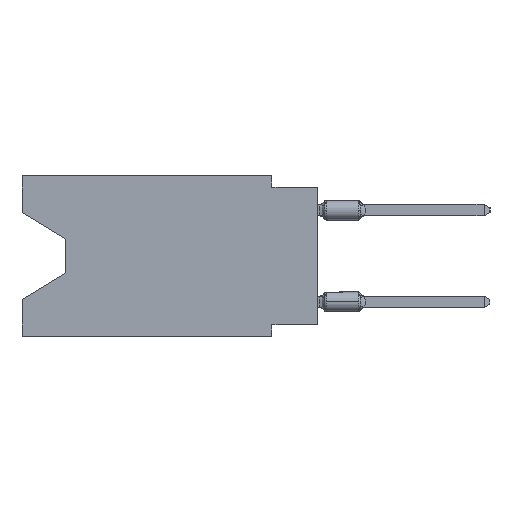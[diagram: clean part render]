
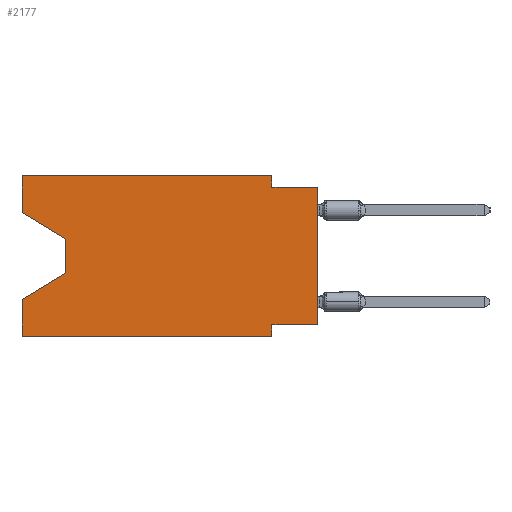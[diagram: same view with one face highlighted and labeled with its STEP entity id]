
A CAD part, left-side view. The second image highlights one B-rep face of the part: STEP entity #2177.
In plain terms, the highlighted planar face has unit normal (-1, 0, 0).
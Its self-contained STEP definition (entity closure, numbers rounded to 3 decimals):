
#264 = LINE ( 'NONE', #4096, #41204 ) ;
#921 = EDGE_CURVE ( 'NONE', #3850, #40693, #20967, .T. ) ;
#2175 = ORIENTED_EDGE ( 'NONE', *, *, #921, .F. ) ;
#2177 = ADVANCED_FACE ( 'NONE', ( #38050 ), #8898, .F. ) ;
#2750 = VERTEX_POINT ( 'NONE', #29670 ) ;
#3200 = CARTESIAN_POINT ( 'NONE',  ( 0., 16.383, 0. ) ) ;
#3461 = DIRECTION ( 'NONE',  ( 0., 0.855, -0.519 ) ) ;
#3782 = CARTESIAN_POINT ( 'NONE',  ( 0., 0., -8.255 ) ) ;
#3817 = LINE ( 'NONE', #3200, #16447 ) ;
#3850 = VERTEX_POINT ( 'NONE', #8228 ) ;
#4074 = ORIENTED_EDGE ( 'NONE', *, *, #18915, .T. ) ;
#4096 = CARTESIAN_POINT ( 'NONE',  ( 0., 0., -0.635 ) ) ;
#4331 = CARTESIAN_POINT ( 'NONE',  ( 0., 2.54, -8.89 ) ) ;
#5029 = VERTEX_POINT ( 'NONE', #3782 ) ;
#5121 = VECTOR ( 'NONE', #6302, 1000. ) ;
#5328 = EDGE_CURVE ( 'NONE', #8839, #17638, #25675, .T. ) ;
#5792 = CARTESIAN_POINT ( 'NONE',  ( 0., 16.383, 0. ) ) ;
#5820 = EDGE_LOOP ( 'NONE', ( #4074, #32551, #6760, #31467, #9528, #18816, #40151, #29738, #10410, #2175, #34779, #16425 ) ) ;
#6302 = DIRECTION ( 'NONE',  ( 0., 0., -1. ) ) ;
#6650 = CARTESIAN_POINT ( 'NONE',  ( 0., 13.97, -5.385 ) ) ;
#6760 = ORIENTED_EDGE ( 'NONE', *, *, #22581, .T. ) ;
#8009 = VECTOR ( 'NONE', #10311, 1000. ) ;
#8228 = CARTESIAN_POINT ( 'NONE',  ( 0., 2.54, 0. ) ) ;
#8285 = EDGE_CURVE ( 'NONE', #5029, #39545, #39004, .T. ) ;
#8588 = LINE ( 'NONE', #41334, #36419 ) ;
#8731 = EDGE_CURVE ( 'NONE', #36822, #3850, #16636, .T. ) ;
#8839 = VERTEX_POINT ( 'NONE', #11073 ) ;
#8898 = PLANE ( 'NONE',  #18575 ) ;
#9528 = ORIENTED_EDGE ( 'NONE', *, *, #11118, .T. ) ;
#9537 = EDGE_CURVE ( 'NONE', #40693, #39545, #264, .T. ) ;
#10311 = DIRECTION ( 'NONE',  ( 0., -1., 0. ) ) ;
#10410 = ORIENTED_EDGE ( 'NONE', *, *, #9537, .F. ) ;
#10954 = CARTESIAN_POINT ( 'NONE',  ( 0., 2.54, 0. ) ) ;
#11073 = CARTESIAN_POINT ( 'NONE',  ( 0., 13.97, -3.505 ) ) ;
#11118 = EDGE_CURVE ( 'NONE', #41125, #34524, #26472, .T. ) ;
#13070 = CARTESIAN_POINT ( 'NONE',  ( 0., 2.54, -8.89 ) ) ;
#13257 = DIRECTION ( 'NONE',  ( 0., -0.855, -0.519 ) ) ;
#13258 = DIRECTION ( 'NONE',  ( 0., 0., 1. ) ) ;
#13309 = VERTEX_POINT ( 'NONE', #18416 ) ;
#13465 = LINE ( 'NONE', #22075, #17119 ) ;
#13531 = VERTEX_POINT ( 'NONE', #40392 ) ;
#14518 = VECTOR ( 'NONE', #38144, 1000. ) ;
#15238 = CARTESIAN_POINT ( 'NONE',  ( 0., 16.383, 0. ) ) ;
#16425 = ORIENTED_EDGE ( 'NONE', *, *, #33007, .F. ) ;
#16447 = VECTOR ( 'NONE', #36173, 1000. ) ;
#16636 = LINE ( 'NONE', #29585, #39109 ) ;
#16873 = CARTESIAN_POINT ( 'NONE',  ( 0., 13.97, -5.385 ) ) ;
#16905 = EDGE_CURVE ( 'NONE', #13309, #34524, #29226, .T. ) ;
#16914 = CARTESIAN_POINT ( 'NONE',  ( 0., 16.383, -8.89 ) ) ;
#17119 = VECTOR ( 'NONE', #13257, 1000. ) ;
#17638 = VERTEX_POINT ( 'NONE', #6650 ) ;
#18416 = CARTESIAN_POINT ( 'NONE',  ( 0., 2.54, -8.255 ) ) ;
#18575 = AXIS2_PLACEMENT_3D ( 'NONE', #27632, #21889, #40596 ) ;
#18816 = ORIENTED_EDGE ( 'NONE', *, *, #16905, .F. ) ;
#18915 = EDGE_CURVE ( 'NONE', #2750, #8839, #13465, .T. ) ;
#20071 = DIRECTION ( 'NONE',  ( 0., -1., 0. ) ) ;
#20967 = LINE ( 'NONE', #10954, #24700 ) ;
#21576 = DIRECTION ( 'NONE',  ( 0., 1., 0. ) ) ;
#21889 = DIRECTION ( 'NONE',  ( 1., 0., 0. ) ) ;
#22075 = CARTESIAN_POINT ( 'NONE',  ( 0., 16.383, -2.038 ) ) ;
#22581 = EDGE_CURVE ( 'NONE', #17638, #13531, #32610, .T. ) ;
#23709 = EDGE_CURVE ( 'NONE', #41125, #13531, #3817, .T. ) ;
#23864 = CARTESIAN_POINT ( 'NONE',  ( 0., 0., -0.635 ) ) ;
#24700 = VECTOR ( 'NONE', #36501, 1000. ) ;
#25161 = LINE ( 'NONE', #5792, #14518 ) ;
#25675 = LINE ( 'NONE', #38649, #5121 ) ;
#26041 = DIRECTION ( 'NONE',  ( 0., 0., -1. ) ) ;
#26392 = DIRECTION ( 'NONE',  ( 0., -1., 0. ) ) ;
#26472 = LINE ( 'NONE', #39458, #8009 ) ;
#26861 = CARTESIAN_POINT ( 'NONE',  ( 0., 0., 0. ) ) ;
#27041 = EDGE_CURVE ( 'NONE', #5029, #13309, #8588, .T. ) ;
#27544 = VECTOR ( 'NONE', #13258, 1000. ) ;
#27632 = CARTESIAN_POINT ( 'NONE',  ( 0., 16.383, 0. ) ) ;
#29221 = VECTOR ( 'NONE', #26041, 1000. ) ;
#29226 = LINE ( 'NONE', #13070, #29221 ) ;
#29585 = CARTESIAN_POINT ( 'NONE',  ( 0., 16.383, 0. ) ) ;
#29670 = CARTESIAN_POINT ( 'NONE',  ( 0., 16.383, -2.038 ) ) ;
#29738 = ORIENTED_EDGE ( 'NONE', *, *, #8285, .T. ) ;
#30562 = CARTESIAN_POINT ( 'NONE',  ( 0., 2.54, -0.635 ) ) ;
#31467 = ORIENTED_EDGE ( 'NONE', *, *, #23709, .F. ) ;
#32551 = ORIENTED_EDGE ( 'NONE', *, *, #5328, .T. ) ;
#32610 = LINE ( 'NONE', #16873, #39438 ) ;
#33007 = EDGE_CURVE ( 'NONE', #2750, #36822, #25161, .T. ) ;
#34524 = VERTEX_POINT ( 'NONE', #4331 ) ;
#34779 = ORIENTED_EDGE ( 'NONE', *, *, #8731, .F. ) ;
#36173 = DIRECTION ( 'NONE',  ( 0., 0., 1. ) ) ;
#36419 = VECTOR ( 'NONE', #21576, 1000. ) ;
#36501 = DIRECTION ( 'NONE',  ( 0., 0., -1. ) ) ;
#36822 = VERTEX_POINT ( 'NONE', #15238 ) ;
#38050 = FACE_OUTER_BOUND ( 'NONE', #5820, .T. ) ;
#38144 = DIRECTION ( 'NONE',  ( 0., 0., 1. ) ) ;
#38649 = CARTESIAN_POINT ( 'NONE',  ( 0., 13.97, -3.505 ) ) ;
#39004 = LINE ( 'NONE', #26861, #27544 ) ;
#39109 = VECTOR ( 'NONE', #26392, 1000. ) ;
#39438 = VECTOR ( 'NONE', #3461, 1000. ) ;
#39458 = CARTESIAN_POINT ( 'NONE',  ( 0., 16.383, -8.89 ) ) ;
#39545 = VERTEX_POINT ( 'NONE', #23864 ) ;
#40151 = ORIENTED_EDGE ( 'NONE', *, *, #27041, .F. ) ;
#40392 = CARTESIAN_POINT ( 'NONE',  ( 0., 16.383, -6.852 ) ) ;
#40596 = DIRECTION ( 'NONE',  ( 0., 0., -1. ) ) ;
#40693 = VERTEX_POINT ( 'NONE', #30562 ) ;
#41125 = VERTEX_POINT ( 'NONE', #16914 ) ;
#41204 = VECTOR ( 'NONE', #20071, 1000. ) ;
#41334 = CARTESIAN_POINT ( 'NONE',  ( 0., 0., -8.255 ) ) ;
